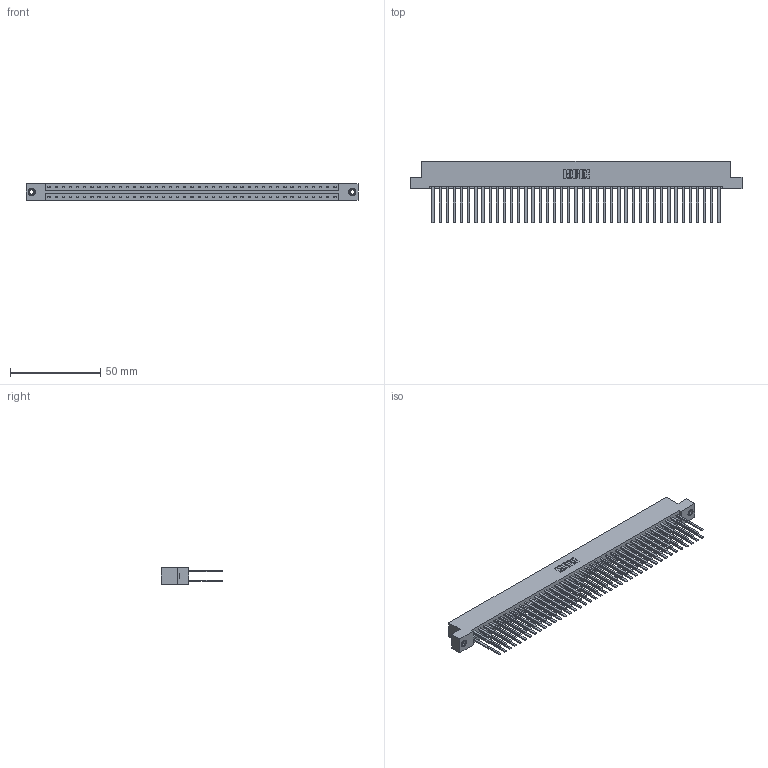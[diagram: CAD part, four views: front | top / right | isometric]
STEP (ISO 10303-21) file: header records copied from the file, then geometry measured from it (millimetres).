
FILE_DESCRIPTION (( 'STEP AP203' ), '1' );
FILE_NAME ('833-082-544-207.STEP', '2020-06-05T23:56:29', ( '' ), ( '' ), 'SwSTEP 2.0', 'SolidWorks 2020', '' );
FILE_SCHEMA (( 'CONFIG_CONTROL_DESIGN' ));
Length unit declared in the file: inch
Products named in the file (4): 833 Part_Flush - .156 Dia - TI; 345-250-001_345-250-005-103; 833-082-544-207; 345-292-001_345-293-144
Assembly tree (85 placements, depth 2):
  833-082-544-207
    833 Part_Flush - .156 Dia - TI
    345-292-001_345-293-144  x82
    345-250-001_345-250-005-103  x2
Bounding box: 184 x 34.3 x 9.4 mm (x, y, z)
Volume: 19911.7 mm3; surface area: 27265.1 mm2
Topology: 85 solids, 85 shells, 3946 faces, 11681 edges, 7670 vertices
Faces by surface type: plane 2726, cylinder 1204, cone 12, torus 4
Entity records: 27508 total; most frequent: CARTESIAN_POINT 4541, ORIENTED_EDGE 4470, DIRECTION 3909, EDGE_CURVE 2235, LINE 2091, VECTOR 2091, VERTEX_POINT 1484, AXIS2_PLACEMENT_3D 909
